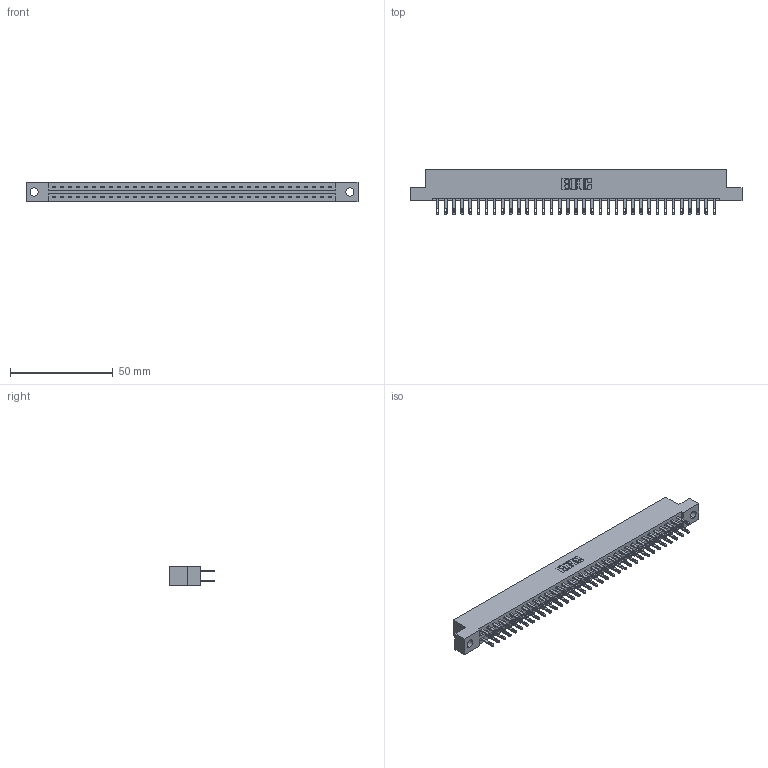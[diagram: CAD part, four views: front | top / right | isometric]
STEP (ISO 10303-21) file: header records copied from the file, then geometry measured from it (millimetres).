
FILE_DESCRIPTION (( 'STEP AP203' ), '1' );
FILE_NAME ('337-070-500-204.STEP', '2019-10-10T00:54:46', ( '' ), ( '' ), 'SwSTEP 2.0', 'SolidWorks 2016', '' );
FILE_SCHEMA (( 'CONFIG_CONTROL_DESIGN' ));
Length unit declared in the file: inch
Products named in the file (3): 337-070-500-204; 337 Part_Flush Mounting Lugs - 0.156 Dia-TH; 345-292-001_345-293-100
Assembly tree (71 placements, depth 2):
  337-070-500-204
    337 Part_Flush Mounting Lugs - 0.156 Dia-TH
    345-292-001_345-293-100  x70
Bounding box: 161.7 x 21.85 x 9.4 mm (x, y, z)
Volume: 17073.7 mm3; surface area: 19808 mm2
Topology: 71 solids, 71 shells, 3614 faces, 11021 edges, 7346 vertices
Faces by surface type: plane 2310, cylinder 1304
Entity records: 27975 total; most frequent: CARTESIAN_POINT 4718, ORIENTED_EDGE 4654, DIRECTION 4027, EDGE_CURVE 2327, LINE 2195, VECTOR 2195, VERTEX_POINT 1550, AXIS2_PLACEMENT_3D 916
